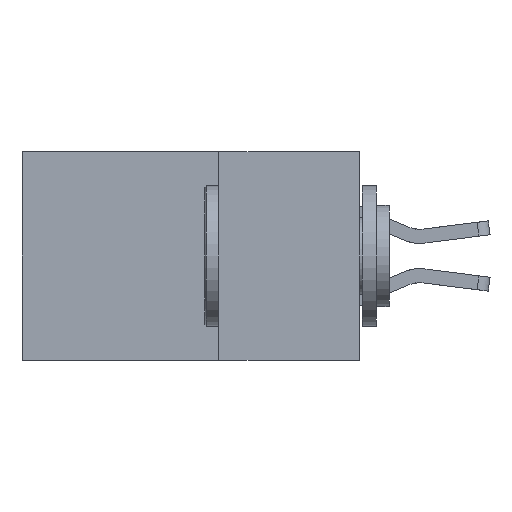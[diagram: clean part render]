
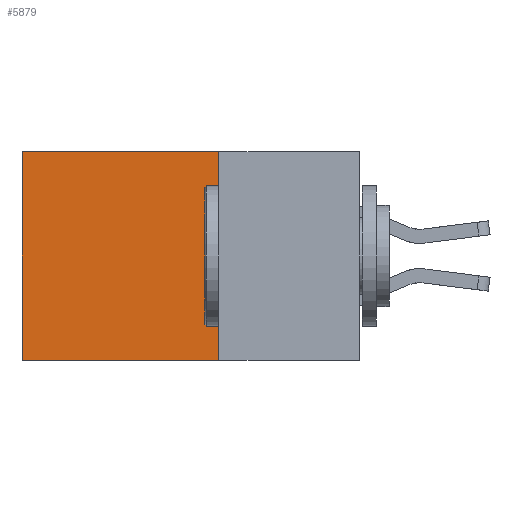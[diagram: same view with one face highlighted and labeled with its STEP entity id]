
A CAD part, left-side view. The second image highlights one B-rep face of the part: STEP entity #5879.
In plain terms, the highlighted planar face has unit normal (-1, 0, 0).
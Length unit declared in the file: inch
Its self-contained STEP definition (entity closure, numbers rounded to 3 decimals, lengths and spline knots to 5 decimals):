
#486 = DIRECTION ( 'NONE',  ( 0., 1., 0. ) ) ;
#498 = CARTESIAN_POINT ( 'NONE',  ( 0.2875, 0.25, 0. ) ) ;
#511 = CARTESIAN_POINT ( 'NONE',  ( 0.2875, 0.25, 0. ) ) ;
#665 = VECTOR ( 'NONE', #6474, 39.37008 ) ;
#694 = DIRECTION ( 'NONE',  ( 0., 0., -1. ) ) ;
#700 = CARTESIAN_POINT ( 'NONE',  ( 0.2875, 0.6, 0. ) ) ;
#790 = VECTOR ( 'NONE', #8634, 39.37008 ) ;
#1147 = AXIS2_PLACEMENT_3D ( 'NONE', #498, #7317, #694 ) ;
#1737 = VECTOR ( 'NONE', #486, 39.37008 ) ;
#2724 = VECTOR ( 'NONE', #3762, 39.37008 ) ;
#2909 = CARTESIAN_POINT ( 'NONE',  ( 0.2875, 0.25, 0. ) ) ;
#2928 = CARTESIAN_POINT ( 'NONE',  ( 0.2875, 0.25, -0.37 ) ) ;
#3113 = ORIENTED_EDGE ( 'NONE', *, *, #5404, .T. ) ;
#3292 = VERTEX_POINT ( 'NONE', #9728 ) ;
#3762 = DIRECTION ( 'NONE',  ( 0., 0., -1. ) ) ;
#3943 = LINE ( 'NONE', #5441, #790 ) ;
#4502 = PLANE ( 'NONE',  #1147 ) ;
#4884 = ORIENTED_EDGE ( 'NONE', *, *, #7731, .F. ) ;
#5404 = EDGE_CURVE ( 'NONE', #8182, #10274, #5516, .T. ) ;
#5441 = CARTESIAN_POINT ( 'NONE',  ( 0.2875, 0.25, -0.37 ) ) ;
#5516 = LINE ( 'NONE', #2909, #1737 ) ;
#5699 = CARTESIAN_POINT ( 'NONE',  ( 0.2875, 0.6, 0. ) ) ;
#5879 = ADVANCED_FACE ( 'NONE', ( #6347 ), #4502, .F. ) ;
#6347 = FACE_OUTER_BOUND ( 'NONE', #9251, .T. ) ;
#6474 = DIRECTION ( 'NONE',  ( 0., 0., -1. ) ) ;
#6989 = EDGE_CURVE ( 'NONE', #10274, #3292, #7137, .T. ) ;
#7137 = LINE ( 'NONE', #5699, #665 ) ;
#7317 = DIRECTION ( 'NONE',  ( 1., 0., 0. ) ) ;
#7496 = ORIENTED_EDGE ( 'NONE', *, *, #7882, .F. ) ;
#7731 = EDGE_CURVE ( 'NONE', #8182, #7932, #9969, .T. ) ;
#7882 = EDGE_CURVE ( 'NONE', #7932, #3292, #3943, .T. ) ;
#7932 = VERTEX_POINT ( 'NONE', #2928 ) ;
#8086 = CARTESIAN_POINT ( 'NONE',  ( 0.2875, 0.25, 0. ) ) ;
#8182 = VERTEX_POINT ( 'NONE', #8086 ) ;
#8634 = DIRECTION ( 'NONE',  ( 0., 1., 0. ) ) ;
#9251 = EDGE_LOOP ( 'NONE', ( #10343, #7496, #4884, #3113 ) ) ;
#9728 = CARTESIAN_POINT ( 'NONE',  ( 0.2875, 0.6, -0.37 ) ) ;
#9969 = LINE ( 'NONE', #511, #2724 ) ;
#10274 = VERTEX_POINT ( 'NONE', #700 ) ;
#10343 = ORIENTED_EDGE ( 'NONE', *, *, #6989, .T. ) ;
